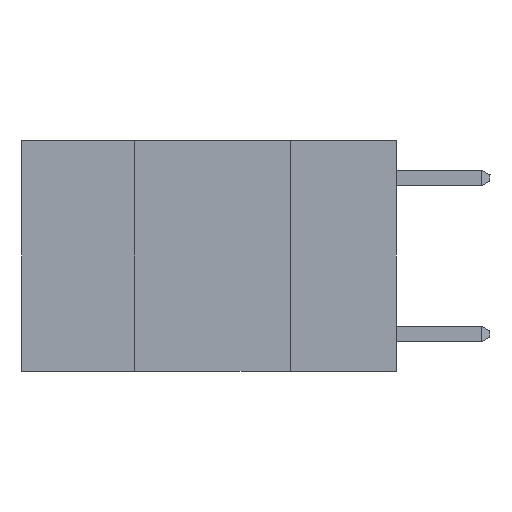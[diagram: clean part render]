
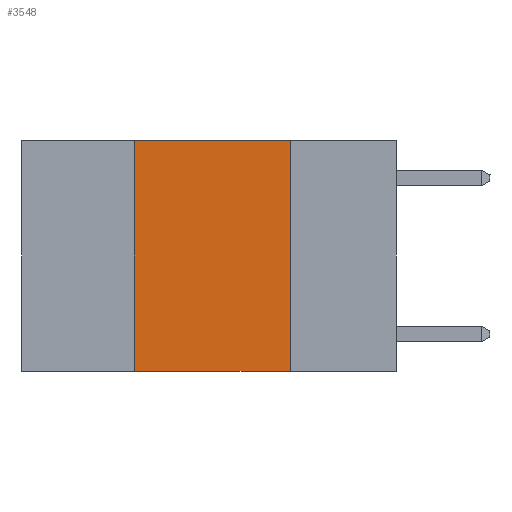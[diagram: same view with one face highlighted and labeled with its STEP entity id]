
A CAD part, left-side view. The second image highlights one B-rep face of the part: STEP entity #3548.
In plain terms, the highlighted planar face has unit normal (-1, 0, 0).
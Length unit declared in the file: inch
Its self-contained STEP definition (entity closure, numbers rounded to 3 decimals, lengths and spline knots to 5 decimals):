
#252 = ORIENTED_EDGE ( 'NONE', *, *, #7735, .F. ) ;
#300 = EDGE_CURVE ( 'NONE', #6331, #9263, #7875, .T. ) ;
#1027 = CARTESIAN_POINT ( 'NONE',  ( 0., 0.6, -0.37 ) ) ;
#1310 = CARTESIAN_POINT ( 'NONE',  ( 0., 0.6, 0. ) ) ;
#1590 = EDGE_CURVE ( 'NONE', #6331, #7740, #5060, .T. ) ;
#1834 = EDGE_CURVE ( 'NONE', #9549, #9263, #2638, .T. ) ;
#2015 = ORIENTED_EDGE ( 'NONE', *, *, #300, .T. ) ;
#2102 = CARTESIAN_POINT ( 'NONE',  ( 0., 0.17, 0. ) ) ;
#2638 = LINE ( 'NONE', #5707, #6013 ) ;
#2722 = DIRECTION ( 'NONE',  ( 0., -1., 0. ) ) ;
#3244 = VECTOR ( 'NONE', #4105, 39.37008 ) ;
#3406 = LINE ( 'NONE', #6482, #6642 ) ;
#3409 = DIRECTION ( 'NONE',  ( 0., 0., -1. ) ) ;
#3548 = ADVANCED_FACE ( 'NONE', ( #8911 ), #8155, .F. ) ;
#3980 = CARTESIAN_POINT ( 'NONE',  ( 0., 0.17, -0.37 ) ) ;
#4105 = DIRECTION ( 'NONE',  ( 0., -1., 0. ) ) ;
#4780 = VECTOR ( 'NONE', #5203, 39.37008 ) ;
#5060 = LINE ( 'NONE', #8981, #4780 ) ;
#5134 = CARTESIAN_POINT ( 'NONE',  ( 0., 0.42, 0. ) ) ;
#5203 = DIRECTION ( 'NONE',  ( 0., 0., 1. ) ) ;
#5215 = CARTESIAN_POINT ( 'NONE',  ( 0., 0.42, -0.37 ) ) ;
#5376 = EDGE_LOOP ( 'NONE', ( #5747, #252, #6248, #2015 ) ) ;
#5707 = CARTESIAN_POINT ( 'NONE',  ( 0., 0.17, 0. ) ) ;
#5747 = ORIENTED_EDGE ( 'NONE', *, *, #1834, .F. ) ;
#6013 = VECTOR ( 'NONE', #8716, 39.37008 ) ;
#6248 = ORIENTED_EDGE ( 'NONE', *, *, #1590, .F. ) ;
#6331 = VERTEX_POINT ( 'NONE', #5215 ) ;
#6482 = CARTESIAN_POINT ( 'NONE',  ( 0., 0.6, 0. ) ) ;
#6485 = DIRECTION ( 'NONE',  ( 1., 0., 0. ) ) ;
#6642 = VECTOR ( 'NONE', #2722, 39.37008 ) ;
#7735 = EDGE_CURVE ( 'NONE', #7740, #9549, #3406, .T. ) ;
#7740 = VERTEX_POINT ( 'NONE', #5134 ) ;
#7875 = LINE ( 'NONE', #1027, #3244 ) ;
#8155 = PLANE ( 'NONE',  #9550 ) ;
#8716 = DIRECTION ( 'NONE',  ( 0., 0., -1. ) ) ;
#8911 = FACE_OUTER_BOUND ( 'NONE', #5376, .T. ) ;
#8981 = CARTESIAN_POINT ( 'NONE',  ( 0., 0.42, 0. ) ) ;
#9263 = VERTEX_POINT ( 'NONE', #3980 ) ;
#9549 = VERTEX_POINT ( 'NONE', #2102 ) ;
#9550 = AXIS2_PLACEMENT_3D ( 'NONE', #1310, #6485, #3409 ) ;
